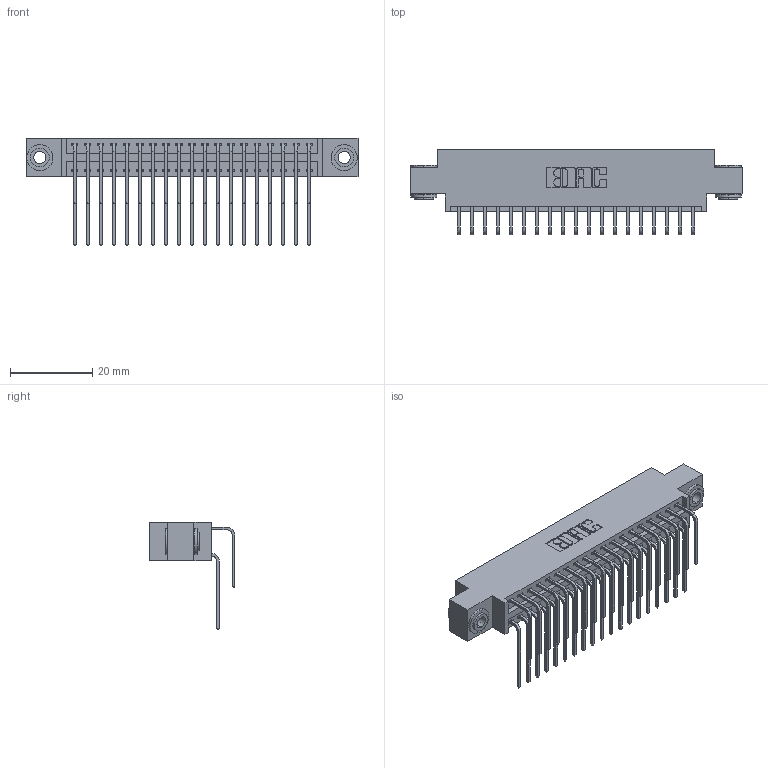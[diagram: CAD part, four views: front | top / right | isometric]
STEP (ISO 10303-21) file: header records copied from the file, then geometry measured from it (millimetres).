
FILE_DESCRIPTION (( 'STEP AP203' ), '1' );
FILE_NAME ('346-038-559-803.STEP', '2022-05-20T00:41:24', ( '' ), ( '' ), 'SwSTEP 2.0', 'SolidWorks 2020', '' );
FILE_SCHEMA (( 'CONFIG_CONTROL_DESIGN' ));
Length unit declared in the file: inch
Products named in the file (5): 345-292-001_558 559 Tail - 1; 346 Part_0.170 Offset - 0.156 Dia-TH; 346-038-559-803; 345-292-001_559 Tail - 2; 345-250-002_345-250-002-102
Assembly tree (41 placements, depth 2):
  346-038-559-803
    346 Part_0.170 Offset - 0.156 Dia-TH
    345-292-001_558 559 Tail - 1  x19
    345-292-001_559 Tail - 2  x19
    345-250-002_345-250-002-102  x2
Bounding box: 80.9 x 20.89 x 26.16 mm (x, y, z)
Volume: 7775.9 mm3; surface area: 11807 mm2
Topology: 41 solids, 41 shells, 2230 faces, 6571 edges, 4326 vertices
Faces by surface type: plane 1510, cylinder 712, cone 8
Entity records: 18478 total; most frequent: CARTESIAN_POINT 3112, ORIENTED_EDGE 2986, DIRECTION 2795, EDGE_CURVE 1493, VECTOR 1221, LINE 1221, VERTEX_POINT 990, AXIS2_PLACEMENT_3D 787
